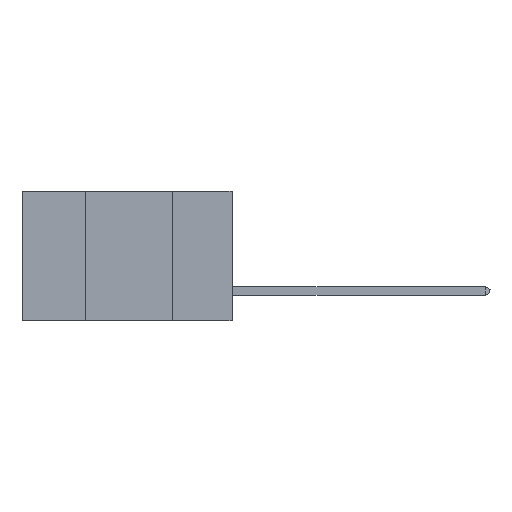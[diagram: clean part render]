
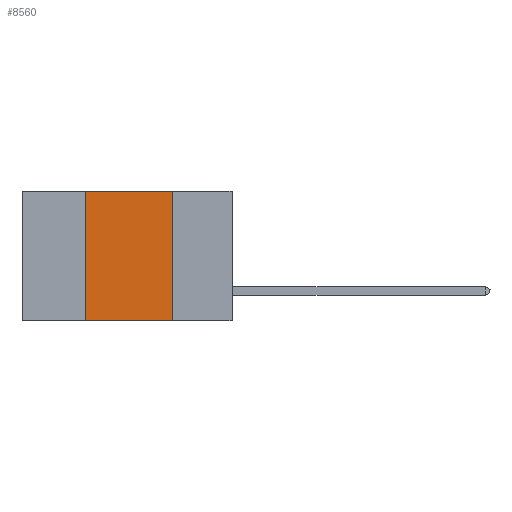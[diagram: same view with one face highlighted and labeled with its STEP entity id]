
A CAD part, left-side view. The second image highlights one B-rep face of the part: STEP entity #8560.
In plain terms, the highlighted planar face has unit normal (-1, 0, 0).
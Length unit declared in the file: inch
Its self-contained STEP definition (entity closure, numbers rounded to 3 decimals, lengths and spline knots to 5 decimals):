
#886 = LINE ( 'NONE', #8735, #11812 ) ;
#1113 = EDGE_LOOP ( 'NONE', ( #9636, #12096, #5115, #24187 ) ) ;
#1428 = VERTEX_POINT ( 'NONE', #20778 ) ;
#1841 = FACE_OUTER_BOUND ( 'NONE', #1113, .T. ) ;
#1982 = CARTESIAN_POINT ( 'NONE',  ( 0., 0.6, 0. ) ) ;
#2036 = CARTESIAN_POINT ( 'NONE',  ( 0., 0.42, 0. ) ) ;
#3419 = DIRECTION ( 'NONE',  ( 0., 0., -1. ) ) ;
#5115 = ORIENTED_EDGE ( 'NONE', *, *, #15790, .F. ) ;
#6493 = CARTESIAN_POINT ( 'NONE',  ( 0., 0.42, 0. ) ) ;
#7192 = DIRECTION ( 'NONE',  ( 0., 0., 1. ) ) ;
#7371 = DIRECTION ( 'NONE',  ( 1., 0., 0. ) ) ;
#8560 = ADVANCED_FACE ( 'NONE', ( #1841 ), #12579, .F. ) ;
#8735 = CARTESIAN_POINT ( 'NONE',  ( 0., 0.17, 0. ) ) ;
#9636 = ORIENTED_EDGE ( 'NONE', *, *, #34303, .F. ) ;
#9961 = VERTEX_POINT ( 'NONE', #31624 ) ;
#11636 = AXIS2_PLACEMENT_3D ( 'NONE', #26098, #7371, #12814 ) ;
#11812 = VECTOR ( 'NONE', #3419, 39.37008 ) ;
#12096 = ORIENTED_EDGE ( 'NONE', *, *, #23603, .F. ) ;
#12579 = PLANE ( 'NONE',  #11636 ) ;
#12814 = DIRECTION ( 'NONE',  ( 0., 0., -1. ) ) ;
#12817 = CARTESIAN_POINT ( 'NONE',  ( 0., 0.6, -0.37 ) ) ;
#13948 = VECTOR ( 'NONE', #7192, 39.37008 ) ;
#15790 = EDGE_CURVE ( 'NONE', #34008, #32512, #17308, .T. ) ;
#17308 = LINE ( 'NONE', #2036, #13948 ) ;
#19982 = CARTESIAN_POINT ( 'NONE',  ( 0., 0.42, -0.37 ) ) ;
#20715 = VECTOR ( 'NONE', #31617, 39.37008 ) ;
#20778 = CARTESIAN_POINT ( 'NONE',  ( 0., 0.17, 0. ) ) ;
#21203 = LINE ( 'NONE', #1982, #32975 ) ;
#23603 = EDGE_CURVE ( 'NONE', #32512, #1428, #21203, .T. ) ;
#24187 = ORIENTED_EDGE ( 'NONE', *, *, #33260, .T. ) ;
#26098 = CARTESIAN_POINT ( 'NONE',  ( 0., 0.6, 0. ) ) ;
#28757 = LINE ( 'NONE', #12817, #20715 ) ;
#31617 = DIRECTION ( 'NONE',  ( 0., -1., 0. ) ) ;
#31624 = CARTESIAN_POINT ( 'NONE',  ( 0., 0.17, -0.37 ) ) ;
#31877 = DIRECTION ( 'NONE',  ( 0., -1., 0. ) ) ;
#32512 = VERTEX_POINT ( 'NONE', #6493 ) ;
#32975 = VECTOR ( 'NONE', #31877, 39.37008 ) ;
#33260 = EDGE_CURVE ( 'NONE', #34008, #9961, #28757, .T. ) ;
#34008 = VERTEX_POINT ( 'NONE', #19982 ) ;
#34303 = EDGE_CURVE ( 'NONE', #1428, #9961, #886, .T. ) ;
